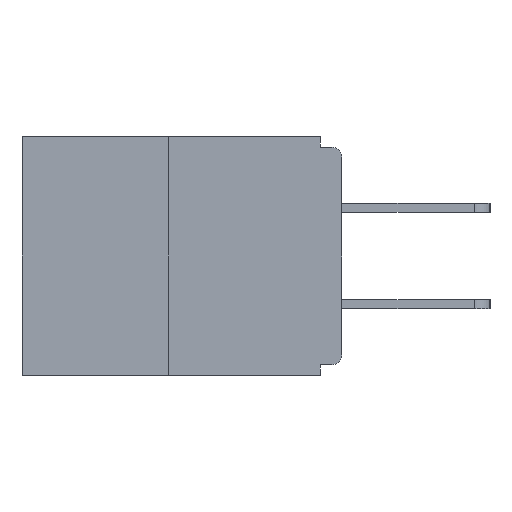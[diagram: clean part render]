
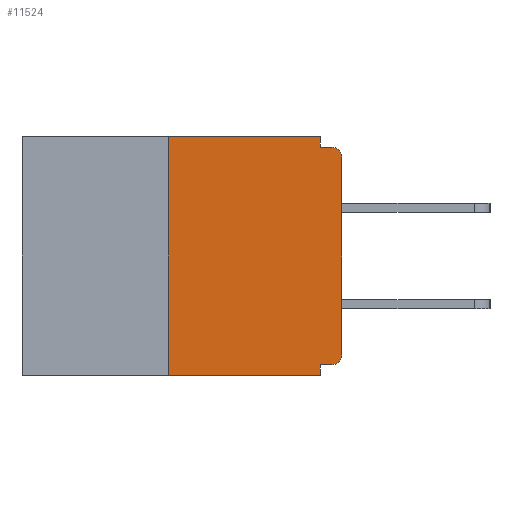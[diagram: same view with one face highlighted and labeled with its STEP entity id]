
A CAD part, left-side view. The second image highlights one B-rep face of the part: STEP entity #11524.
In plain terms, the highlighted planar face has unit normal (-1, 0, 0).
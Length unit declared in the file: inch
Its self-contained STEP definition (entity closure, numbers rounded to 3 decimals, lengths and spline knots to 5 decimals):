
#92 = ORIENTED_EDGE ( 'NONE', *, *, #19252, .T. ) ;
#344 = ORIENTED_EDGE ( 'NONE', *, *, #20351, .T. ) ;
#633 = CARTESIAN_POINT ( 'NONE',  ( 0., 0.031, -0.343 ) ) ;
#1360 = ORIENTED_EDGE ( 'NONE', *, *, #9498, .T. ) ;
#1537 = EDGE_CURVE ( 'NONE', #2962, #5714, #1612, .T. ) ;
#1612 = LINE ( 'NONE', #9353, #18438 ) ;
#1681 = CARTESIAN_POINT ( 'NONE',  ( 0., 0.031, 0. ) ) ;
#2559 = VECTOR ( 'NONE', #13520, 39.37008 ) ;
#2601 = CARTESIAN_POINT ( 'NONE',  ( 0., 0.031, 0. ) ) ;
#2835 = ORIENTED_EDGE ( 'NONE', *, *, #1537, .F. ) ;
#2962 = VERTEX_POINT ( 'NONE', #23534 ) ;
#3067 = LINE ( 'NONE', #18138, #16436 ) ;
#3635 = CARTESIAN_POINT ( 'NONE',  ( 0., 0.015, -0.03 ) ) ;
#4778 = CARTESIAN_POINT ( 'NONE',  ( 0., 0., -0.015 ) ) ;
#4956 = DIRECTION ( 'NONE',  ( 0., 0., 1. ) ) ;
#5117 = CARTESIAN_POINT ( 'NONE',  ( 0., 0., -0.313 ) ) ;
#5258 = EDGE_CURVE ( 'NONE', #5714, #12376, #15917, .T. ) ;
#5683 = LINE ( 'NONE', #19121, #2559 ) ;
#5714 = VERTEX_POINT ( 'NONE', #1681 ) ;
#6465 = ORIENTED_EDGE ( 'NONE', *, *, #15003, .F. ) ;
#6664 = VECTOR ( 'NONE', #24188, 39.37008 ) ;
#7252 = CARTESIAN_POINT ( 'NONE',  ( 0., 0.25, 0. ) ) ;
#7577 = ORIENTED_EDGE ( 'NONE', *, *, #17956, .F. ) ;
#7677 = AXIS2_PLACEMENT_3D ( 'NONE', #23736, #10520, #21734 ) ;
#7692 = CARTESIAN_POINT ( 'NONE',  ( 0., 0.031, -0.328 ) ) ;
#7979 = CARTESIAN_POINT ( 'NONE',  ( 0., 0.015, -0.015 ) ) ;
#8160 = FACE_OUTER_BOUND ( 'NONE', #15038, .T. ) ;
#8166 = EDGE_CURVE ( 'NONE', #14699, #11070, #22008, .T. ) ;
#8197 = CARTESIAN_POINT ( 'NONE',  ( 0., 0.031, -0.343 ) ) ;
#8797 = CARTESIAN_POINT ( 'NONE',  ( 0., 0.031, -0.015 ) ) ;
#9107 = DIRECTION ( 'NONE',  ( 0., 0., -1. ) ) ;
#9178 = CIRCLE ( 'NONE', #11579, 0.015 ) ;
#9350 = LINE ( 'NONE', #7252, #6664 ) ;
#9353 = CARTESIAN_POINT ( 'NONE',  ( 0., 0.46, 0. ) ) ;
#9498 = EDGE_CURVE ( 'NONE', #19792, #20744, #9178, .T. ) ;
#10520 = DIRECTION ( 'NONE',  ( 1., 0., 0. ) ) ;
#10768 = LINE ( 'NONE', #16907, #17206 ) ;
#11070 = VERTEX_POINT ( 'NONE', #5117 ) ;
#11264 = AXIS2_PLACEMENT_3D ( 'NONE', #12484, #24457, #9107 ) ;
#11524 = ADVANCED_FACE ( 'NONE', ( #8160 ), #17623, .F. ) ;
#11579 = AXIS2_PLACEMENT_3D ( 'NONE', #3635, #18585, #22832 ) ;
#12246 = DIRECTION ( 'NONE',  ( 0., -1., 0. ) ) ;
#12376 = VERTEX_POINT ( 'NONE', #8797 ) ;
#12484 = CARTESIAN_POINT ( 'NONE',  ( 0., 0.015, -0.313 ) ) ;
#13520 = DIRECTION ( 'NONE',  ( 0., -1., 0. ) ) ;
#13656 = EDGE_CURVE ( 'NONE', #21874, #2962, #9350, .T. ) ;
#14115 = LINE ( 'NONE', #4778, #17517 ) ;
#14614 = ORIENTED_EDGE ( 'NONE', *, *, #23932, .F. ) ;
#14699 = VERTEX_POINT ( 'NONE', #19957 ) ;
#15003 = EDGE_CURVE ( 'NONE', #22537, #24262, #21161, .T. ) ;
#15038 = EDGE_LOOP ( 'NONE', ( #2835, #19128, #344, #6465, #7577, #22507, #92, #1360, #14614, #23552 ) ) ;
#15917 = LINE ( 'NONE', #2601, #18845 ) ;
#16436 = VECTOR ( 'NONE', #4956, 39.37008 ) ;
#16907 = CARTESIAN_POINT ( 'NONE',  ( 0., 0., -0.328 ) ) ;
#17056 = CARTESIAN_POINT ( 'NONE',  ( 0., 0., -0.03 ) ) ;
#17206 = VECTOR ( 'NONE', #24388, 39.37008 ) ;
#17517 = VECTOR ( 'NONE', #12246, 39.37008 ) ;
#17623 = PLANE ( 'NONE',  #7677 ) ;
#17956 = EDGE_CURVE ( 'NONE', #14699, #22537, #10768, .T. ) ;
#18138 = CARTESIAN_POINT ( 'NONE',  ( 0., 0., 0. ) ) ;
#18438 = VECTOR ( 'NONE', #22551, 39.37008 ) ;
#18585 = DIRECTION ( 'NONE',  ( -1., 0., 0. ) ) ;
#18845 = VECTOR ( 'NONE', #21534, 39.37008 ) ;
#19121 = CARTESIAN_POINT ( 'NONE',  ( 0., 0.46, -0.343 ) ) ;
#19128 = ORIENTED_EDGE ( 'NONE', *, *, #13656, .F. ) ;
#19252 = EDGE_CURVE ( 'NONE', #11070, #19792, #3067, .T. ) ;
#19792 = VERTEX_POINT ( 'NONE', #17056 ) ;
#19957 = CARTESIAN_POINT ( 'NONE',  ( 0., 0.015, -0.328 ) ) ;
#20325 = VECTOR ( 'NONE', #20701, 39.37008 ) ;
#20351 = EDGE_CURVE ( 'NONE', #21874, #24262, #5683, .T. ) ;
#20701 = DIRECTION ( 'NONE',  ( 0., 0., -1. ) ) ;
#20744 = VERTEX_POINT ( 'NONE', #7979 ) ;
#21161 = LINE ( 'NONE', #8197, #20325 ) ;
#21534 = DIRECTION ( 'NONE',  ( 0., 0., -1. ) ) ;
#21734 = DIRECTION ( 'NONE',  ( 0., 0., -1. ) ) ;
#21874 = VERTEX_POINT ( 'NONE', #23347 ) ;
#22008 = CIRCLE ( 'NONE', #11264, 0.015 ) ;
#22507 = ORIENTED_EDGE ( 'NONE', *, *, #8166, .T. ) ;
#22537 = VERTEX_POINT ( 'NONE', #7692 ) ;
#22551 = DIRECTION ( 'NONE',  ( 0., -1., 0. ) ) ;
#22832 = DIRECTION ( 'NONE',  ( 0., 0., -1. ) ) ;
#23347 = CARTESIAN_POINT ( 'NONE',  ( 0., 0.25, -0.343 ) ) ;
#23534 = CARTESIAN_POINT ( 'NONE',  ( 0., 0.25, 0. ) ) ;
#23552 = ORIENTED_EDGE ( 'NONE', *, *, #5258, .F. ) ;
#23736 = CARTESIAN_POINT ( 'NONE',  ( 0., 0.46, 0. ) ) ;
#23932 = EDGE_CURVE ( 'NONE', #12376, #20744, #14115, .T. ) ;
#24188 = DIRECTION ( 'NONE',  ( 0., 0., 1. ) ) ;
#24262 = VERTEX_POINT ( 'NONE', #633 ) ;
#24388 = DIRECTION ( 'NONE',  ( 0., 1., 0. ) ) ;
#24457 = DIRECTION ( 'NONE',  ( -1., 0., 0. ) ) ;
